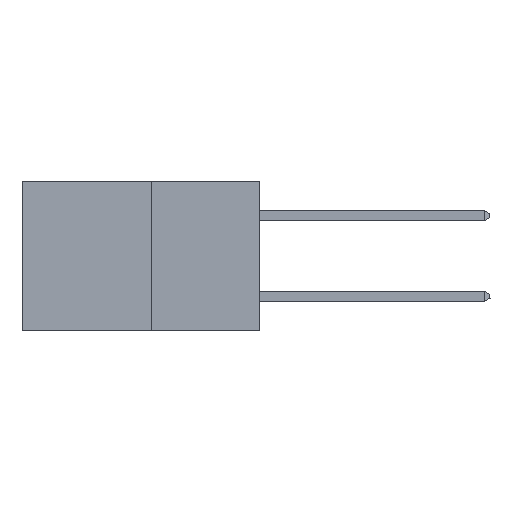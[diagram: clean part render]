
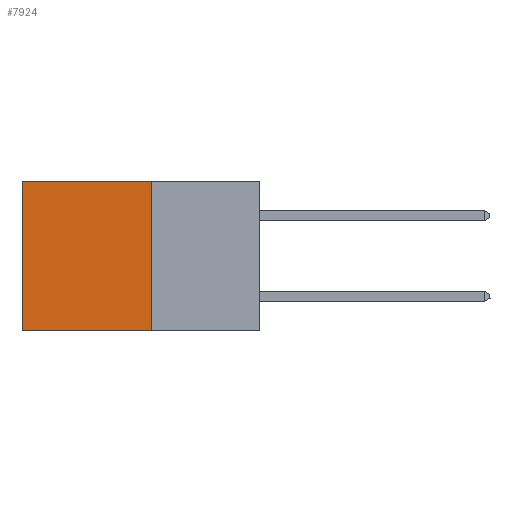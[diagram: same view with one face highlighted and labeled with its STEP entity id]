
A CAD part, left-side view. The second image highlights one B-rep face of the part: STEP entity #7924.
In plain terms, the highlighted planar face has unit normal (-1, 0, 0).
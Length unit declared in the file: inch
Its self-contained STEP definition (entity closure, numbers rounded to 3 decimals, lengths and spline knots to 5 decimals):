
#58 = EDGE_CURVE ( 'NONE', #11901, #5134, #8800, .T. ) ;
#1206 = CARTESIAN_POINT ( 'NONE',  ( 0.277, 0.27, -0.37 ) ) ;
#2706 = DIRECTION ( 'NONE',  ( 0., 0., -1. ) ) ;
#3140 = DIRECTION ( 'NONE',  ( 0., 0., -1. ) ) ;
#4145 = CARTESIAN_POINT ( 'NONE',  ( 0.277, 0.27, 0. ) ) ;
#4331 = VECTOR ( 'NONE', #3140, 39.37008 ) ;
#4479 = FACE_OUTER_BOUND ( 'NONE', #7649, .T. ) ;
#5134 = VERTEX_POINT ( 'NONE', #15163 ) ;
#6032 = CARTESIAN_POINT ( 'NONE',  ( 0.277, 0.27, 0. ) ) ;
#6184 = EDGE_CURVE ( 'NONE', #8037, #10123, #13577, .T. ) ;
#6548 = LINE ( 'NONE', #6032, #7258 ) ;
#6658 = CARTESIAN_POINT ( 'NONE',  ( 0.277, 0.27, -0.37 ) ) ;
#7181 = ORIENTED_EDGE ( 'NONE', *, *, #11833, .F. ) ;
#7258 = VECTOR ( 'NONE', #14144, 39.37008 ) ;
#7276 = AXIS2_PLACEMENT_3D ( 'NONE', #7405, #9646, #2706 ) ;
#7335 = CARTESIAN_POINT ( 'NONE',  ( 0.277, 0.59, 0. ) ) ;
#7405 = CARTESIAN_POINT ( 'NONE',  ( 0.277, 0.27, -0.37 ) ) ;
#7649 = EDGE_LOOP ( 'NONE', ( #9809, #7181, #7876, #14463 ) ) ;
#7876 = ORIENTED_EDGE ( 'NONE', *, *, #6184, .F. ) ;
#7924 = ADVANCED_FACE ( 'NONE', ( #4479 ), #14373, .F. ) ;
#8037 = VERTEX_POINT ( 'NONE', #4145 ) ;
#8314 = DIRECTION ( 'NONE',  ( 0., 1., 0. ) ) ;
#8800 = LINE ( 'NONE', #11706, #12645 ) ;
#9539 = LINE ( 'NONE', #1206, #12332 ) ;
#9646 = DIRECTION ( 'NONE',  ( 1., 0., 0. ) ) ;
#9809 = ORIENTED_EDGE ( 'NONE', *, *, #58, .T. ) ;
#10123 = VERTEX_POINT ( 'NONE', #12328 ) ;
#11706 = CARTESIAN_POINT ( 'NONE',  ( 0.277, 0.59, -0.37 ) ) ;
#11828 = EDGE_CURVE ( 'NONE', #8037, #11901, #6548, .T. ) ;
#11833 = EDGE_CURVE ( 'NONE', #10123, #5134, #9539, .T. ) ;
#11901 = VERTEX_POINT ( 'NONE', #7335 ) ;
#12286 = DIRECTION ( 'NONE',  ( 0., 0., -1. ) ) ;
#12328 = CARTESIAN_POINT ( 'NONE',  ( 0.277, 0.27, -0.37 ) ) ;
#12332 = VECTOR ( 'NONE', #8314, 39.37008 ) ;
#12645 = VECTOR ( 'NONE', #12286, 39.37008 ) ;
#13577 = LINE ( 'NONE', #6658, #4331 ) ;
#14144 = DIRECTION ( 'NONE',  ( 0., 1., 0. ) ) ;
#14373 = PLANE ( 'NONE',  #7276 ) ;
#14463 = ORIENTED_EDGE ( 'NONE', *, *, #11828, .T. ) ;
#15163 = CARTESIAN_POINT ( 'NONE',  ( 0.277, 0.59, -0.37 ) ) ;
